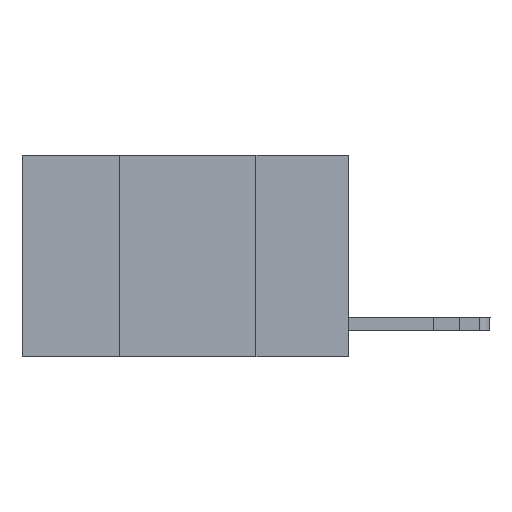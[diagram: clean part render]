
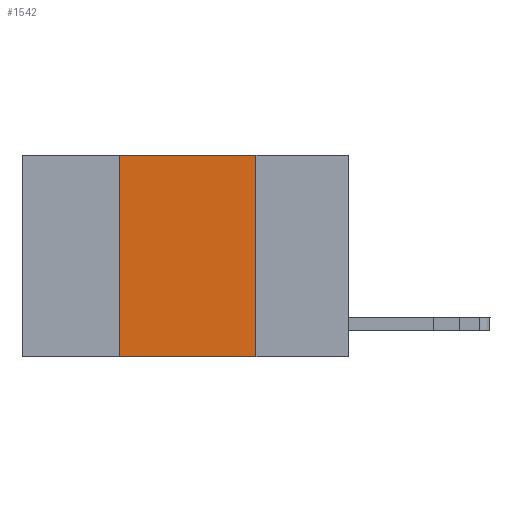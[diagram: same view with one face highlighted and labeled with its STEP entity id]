
A CAD part, left-side view. The second image highlights one B-rep face of the part: STEP entity #1542.
In plain terms, the highlighted planar face has unit normal (-1, 0, 0).
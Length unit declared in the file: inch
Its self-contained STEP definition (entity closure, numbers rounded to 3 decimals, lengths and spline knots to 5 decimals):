
#957 = CARTESIAN_POINT ( 'NONE',  ( 0., 0.42, 0. ) ) ;
#1287 = LINE ( 'NONE', #13286, #5101 ) ;
#1489 = ORIENTED_EDGE ( 'NONE', *, *, #18153, .F. ) ;
#1542 = ADVANCED_FACE ( 'NONE', ( #11834 ), #14345, .F. ) ;
#2169 = EDGE_CURVE ( 'NONE', #5248, #14584, #16134, .T. ) ;
#2617 = AXIS2_PLACEMENT_3D ( 'NONE', #19414, #3443, #12967 ) ;
#2786 = DIRECTION ( 'NONE',  ( 0., -1., 0. ) ) ;
#2857 = CARTESIAN_POINT ( 'NONE',  ( 0., 0.17, -0.37 ) ) ;
#3087 = EDGE_LOOP ( 'NONE', ( #13145, #1489, #16994, #10480 ) ) ;
#3443 = DIRECTION ( 'NONE',  ( 1., 0., 0. ) ) ;
#3598 = VECTOR ( 'NONE', #2786, 39.37008 ) ;
#3673 = VERTEX_POINT ( 'NONE', #2857 ) ;
#5101 = VECTOR ( 'NONE', #10265, 39.37008 ) ;
#5248 = VERTEX_POINT ( 'NONE', #10687 ) ;
#5750 = VERTEX_POINT ( 'NONE', #6118 ) ;
#5766 = DIRECTION ( 'NONE',  ( 0., 0., 1. ) ) ;
#6038 = LINE ( 'NONE', #12337, #6531 ) ;
#6118 = CARTESIAN_POINT ( 'NONE',  ( 0., 0.17, 0. ) ) ;
#6531 = VECTOR ( 'NONE', #7844, 39.37008 ) ;
#7844 = DIRECTION ( 'NONE',  ( 0., -1., 0. ) ) ;
#8793 = VECTOR ( 'NONE', #5766, 39.37008 ) ;
#10265 = DIRECTION ( 'NONE',  ( 0., 0., -1. ) ) ;
#10480 = ORIENTED_EDGE ( 'NONE', *, *, #18828, .T. ) ;
#10687 = CARTESIAN_POINT ( 'NONE',  ( 0., 0.42, -0.37 ) ) ;
#11834 = FACE_OUTER_BOUND ( 'NONE', #3087, .T. ) ;
#12194 = LINE ( 'NONE', #19335, #3598 ) ;
#12337 = CARTESIAN_POINT ( 'NONE',  ( 0., 0.6, -0.37 ) ) ;
#12967 = DIRECTION ( 'NONE',  ( 0., 0., -1. ) ) ;
#13145 = ORIENTED_EDGE ( 'NONE', *, *, #18094, .F. ) ;
#13286 = CARTESIAN_POINT ( 'NONE',  ( 0., 0.17, 0. ) ) ;
#14345 = PLANE ( 'NONE',  #2617 ) ;
#14584 = VERTEX_POINT ( 'NONE', #19214 ) ;
#16134 = LINE ( 'NONE', #957, #8793 ) ;
#16994 = ORIENTED_EDGE ( 'NONE', *, *, #2169, .F. ) ;
#18094 = EDGE_CURVE ( 'NONE', #5750, #3673, #1287, .T. ) ;
#18153 = EDGE_CURVE ( 'NONE', #14584, #5750, #12194, .T. ) ;
#18828 = EDGE_CURVE ( 'NONE', #5248, #3673, #6038, .T. ) ;
#19214 = CARTESIAN_POINT ( 'NONE',  ( 0., 0.42, 0. ) ) ;
#19335 = CARTESIAN_POINT ( 'NONE',  ( 0., 0.6, 0. ) ) ;
#19414 = CARTESIAN_POINT ( 'NONE',  ( 0., 0.6, 0. ) ) ;
